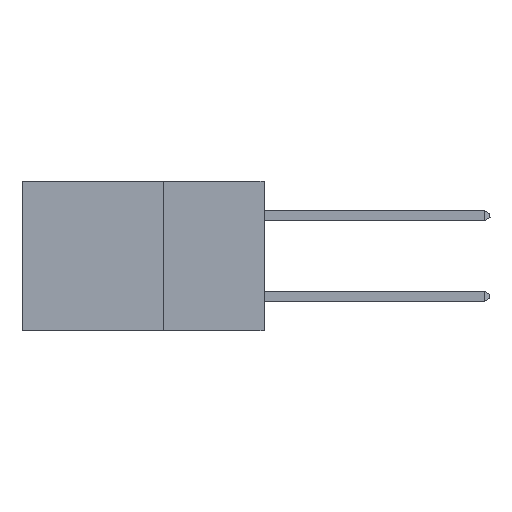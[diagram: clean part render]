
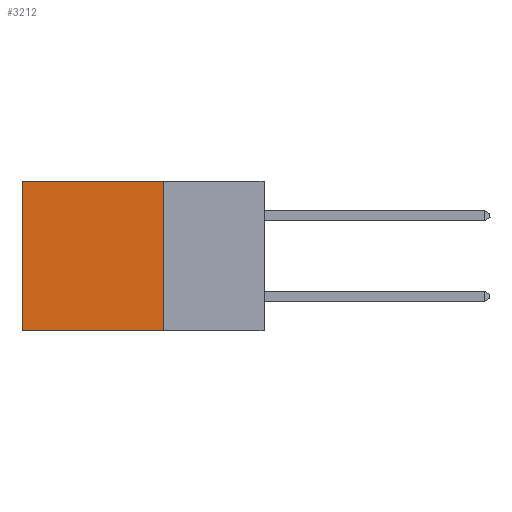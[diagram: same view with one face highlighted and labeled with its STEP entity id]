
A CAD part, left-side view. The second image highlights one B-rep face of the part: STEP entity #3212.
In plain terms, the highlighted planar face has unit normal (-1, 0, 0).
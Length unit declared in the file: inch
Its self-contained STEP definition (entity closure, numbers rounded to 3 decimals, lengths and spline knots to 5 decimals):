
#87 = VERTEX_POINT ( 'NONE', #7104 ) ;
#93 = EDGE_CURVE ( 'NONE', #12215, #87, #1597, .T. ) ;
#1474 = CARTESIAN_POINT ( 'NONE',  ( 0.298, 0.25, -0.37 ) ) ;
#1597 = LINE ( 'NONE', #13218, #11007 ) ;
#1806 = ORIENTED_EDGE ( 'NONE', *, *, #5467, .F. ) ;
#3212 = ADVANCED_FACE ( 'NONE', ( #13153 ), #10633, .F. ) ;
#3332 = VECTOR ( 'NONE', #3393, 39.37008 ) ;
#3393 = DIRECTION ( 'NONE',  ( 0., 0., -1. ) ) ;
#3766 = EDGE_CURVE ( 'NONE', #11806, #4165, #5428, .T. ) ;
#3791 = VECTOR ( 'NONE', #10194, 39.37008 ) ;
#3874 = DIRECTION ( 'NONE',  ( 0., 0., -1. ) ) ;
#4165 = VERTEX_POINT ( 'NONE', #8806 ) ;
#4378 = CARTESIAN_POINT ( 'NONE',  ( 0.298, 0.6, 0. ) ) ;
#4584 = EDGE_CURVE ( 'NONE', #4165, #87, #4601, .T. ) ;
#4601 = LINE ( 'NONE', #4378, #3332 ) ;
#4628 = CARTESIAN_POINT ( 'NONE',  ( 0.298, 0.25, 0. ) ) ;
#4726 = CARTESIAN_POINT ( 'NONE',  ( 0.298, 0.25, 0. ) ) ;
#5386 = VECTOR ( 'NONE', #3874, 39.37008 ) ;
#5428 = LINE ( 'NONE', #12354, #3791 ) ;
#5467 = EDGE_CURVE ( 'NONE', #11806, #12215, #11754, .T. ) ;
#5803 = ORIENTED_EDGE ( 'NONE', *, *, #4584, .T. ) ;
#6165 = DIRECTION ( 'NONE',  ( 0., 1., 0. ) ) ;
#7104 = CARTESIAN_POINT ( 'NONE',  ( 0.298, 0.6, -0.37 ) ) ;
#7588 = CARTESIAN_POINT ( 'NONE',  ( 0.298, 0.25, 0. ) ) ;
#7945 = EDGE_LOOP ( 'NONE', ( #5803, #8389, #1806, #11980 ) ) ;
#8389 = ORIENTED_EDGE ( 'NONE', *, *, #93, .F. ) ;
#8806 = CARTESIAN_POINT ( 'NONE',  ( 0.298, 0.6, 0. ) ) ;
#9546 = AXIS2_PLACEMENT_3D ( 'NONE', #4628, #9735, #12791 ) ;
#9735 = DIRECTION ( 'NONE',  ( 1., 0., 0. ) ) ;
#10194 = DIRECTION ( 'NONE',  ( 0., 1., 0. ) ) ;
#10633 = PLANE ( 'NONE',  #9546 ) ;
#11007 = VECTOR ( 'NONE', #6165, 39.37008 ) ;
#11754 = LINE ( 'NONE', #4726, #5386 ) ;
#11806 = VERTEX_POINT ( 'NONE', #7588 ) ;
#11980 = ORIENTED_EDGE ( 'NONE', *, *, #3766, .T. ) ;
#12215 = VERTEX_POINT ( 'NONE', #1474 ) ;
#12354 = CARTESIAN_POINT ( 'NONE',  ( 0.298, 0.25, 0. ) ) ;
#12791 = DIRECTION ( 'NONE',  ( 0., 0., -1. ) ) ;
#13153 = FACE_OUTER_BOUND ( 'NONE', #7945, .T. ) ;
#13218 = CARTESIAN_POINT ( 'NONE',  ( 0.298, 0.25, -0.37 ) ) ;
